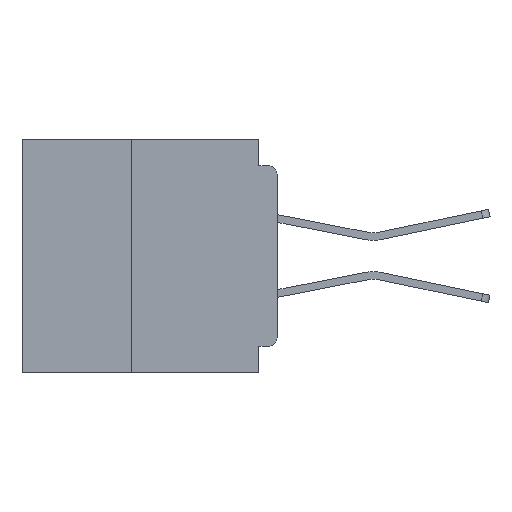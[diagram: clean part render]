
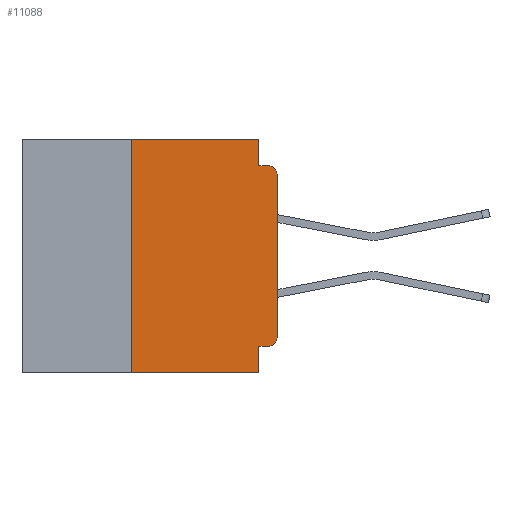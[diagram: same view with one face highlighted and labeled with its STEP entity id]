
A CAD part, left-side view. The second image highlights one B-rep face of the part: STEP entity #11088.
In plain terms, the highlighted planar face has unit normal (-1, 0, 0).
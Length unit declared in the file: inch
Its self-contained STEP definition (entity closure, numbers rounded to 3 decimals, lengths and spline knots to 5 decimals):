
#416 = VECTOR ( 'NONE', #36442, 39.37008 ) ;
#723 = ORIENTED_EDGE ( 'NONE', *, *, #28216, .F. ) ;
#1905 = VECTOR ( 'NONE', #16392, 39.37008 ) ;
#2743 = CARTESIAN_POINT ( 'NONE',  ( 0., 0., -0.06 ) ) ;
#3767 = VERTEX_POINT ( 'NONE', #39235 ) ;
#3960 = LINE ( 'NONE', #8334, #25589 ) ;
#4336 = AXIS2_PLACEMENT_3D ( 'NONE', #12253, #34526, #15499 ) ;
#4358 = EDGE_CURVE ( 'NONE', #33013, #12814, #26104, .T. ) ;
#5211 = CARTESIAN_POINT ( 'NONE',  ( 0., 0.031, -0.045 ) ) ;
#5717 = EDGE_CURVE ( 'NONE', #39130, #32010, #34941, .T. ) ;
#6209 = DIRECTION ( 'NONE',  ( -1., 0., 0. ) ) ;
#6236 = FACE_OUTER_BOUND ( 'NONE', #22828, .T. ) ;
#6773 = DIRECTION ( 'NONE',  ( 0., -1., 0. ) ) ;
#6792 = CARTESIAN_POINT ( 'NONE',  ( 0., 0.031, 0. ) ) ;
#6910 = CARTESIAN_POINT ( 'NONE',  ( 0., 0., -0.355 ) ) ;
#6939 = DIRECTION ( 'NONE',  ( 0., 0., -1. ) ) ;
#7150 = CARTESIAN_POINT ( 'NONE',  ( 0., 0.031, 0. ) ) ;
#7178 = ORIENTED_EDGE ( 'NONE', *, *, #34622, .F. ) ;
#7690 = VECTOR ( 'NONE', #29350, 39.37008 ) ;
#8334 = CARTESIAN_POINT ( 'NONE',  ( 0., 0., 0. ) ) ;
#8445 = VERTEX_POINT ( 'NONE', #33562 ) ;
#9411 = ORIENTED_EDGE ( 'NONE', *, *, #15265, .F. ) ;
#10151 = LINE ( 'NONE', #35265, #41008 ) ;
#10516 = CARTESIAN_POINT ( 'NONE',  ( 0., 0.031, -0.4 ) ) ;
#10726 = VECTOR ( 'NONE', #38511, 39.37008 ) ;
#11088 = ADVANCED_FACE ( 'NONE', ( #6236 ), #16538, .F. ) ;
#12033 = ORIENTED_EDGE ( 'NONE', *, *, #33776, .T. ) ;
#12253 = CARTESIAN_POINT ( 'NONE',  ( 0., 0.015, -0.06 ) ) ;
#12814 = VERTEX_POINT ( 'NONE', #13329 ) ;
#13329 = CARTESIAN_POINT ( 'NONE',  ( 0., 0.25, 0. ) ) ;
#13517 = DIRECTION ( 'NONE',  ( 0., -1., 0. ) ) ;
#14062 = CARTESIAN_POINT ( 'NONE',  ( 0., 0.25, -0.4 ) ) ;
#14987 = ORIENTED_EDGE ( 'NONE', *, *, #4358, .F. ) ;
#15265 = EDGE_CURVE ( 'NONE', #12814, #39130, #19229, .T. ) ;
#15499 = DIRECTION ( 'NONE',  ( 0., 0., -1. ) ) ;
#15989 = LINE ( 'NONE', #16206, #23517 ) ;
#16206 = CARTESIAN_POINT ( 'NONE',  ( 0., 0.031, -0.4 ) ) ;
#16341 = DIRECTION ( 'NONE',  ( 0., 0., -1. ) ) ;
#16392 = DIRECTION ( 'NONE',  ( 0., 0., -1. ) ) ;
#16538 = PLANE ( 'NONE',  #23182 ) ;
#17288 = LINE ( 'NONE', #6910, #7690 ) ;
#17349 = VERTEX_POINT ( 'NONE', #34319 ) ;
#19229 = LINE ( 'NONE', #35338, #10726 ) ;
#20596 = CARTESIAN_POINT ( 'NONE',  ( 0., 0.25, -0.4 ) ) ;
#21818 = CARTESIAN_POINT ( 'NONE',  ( 0., 0., -0.34 ) ) ;
#22828 = EDGE_LOOP ( 'NONE', ( #12033, #38961, #723, #23902, #9411, #14987, #37861, #7178, #33308, #24567 ) ) ;
#22988 = CARTESIAN_POINT ( 'NONE',  ( 0., 0.437, 0. ) ) ;
#23100 = EDGE_CURVE ( 'NONE', #17349, #27999, #38564, .T. ) ;
#23182 = AXIS2_PLACEMENT_3D ( 'NONE', #22988, #26183, #6939 ) ;
#23228 = EDGE_CURVE ( 'NONE', #33013, #26997, #10151, .T. ) ;
#23517 = VECTOR ( 'NONE', #16341, 39.37008 ) ;
#23902 = ORIENTED_EDGE ( 'NONE', *, *, #5717, .F. ) ;
#24482 = CIRCLE ( 'NONE', #4336, 0.015 ) ;
#24567 = ORIENTED_EDGE ( 'NONE', *, *, #23100, .T. ) ;
#25474 = CARTESIAN_POINT ( 'NONE',  ( 0., 0.015, -0.34 ) ) ;
#25589 = VECTOR ( 'NONE', #36937, 39.37008 ) ;
#26104 = LINE ( 'NONE', #14062, #416 ) ;
#26183 = DIRECTION ( 'NONE',  ( 1., 0., 0. ) ) ;
#26702 = VERTEX_POINT ( 'NONE', #2743 ) ;
#26997 = VERTEX_POINT ( 'NONE', #10516 ) ;
#27999 = VERTEX_POINT ( 'NONE', #21818 ) ;
#28181 = VECTOR ( 'NONE', #13517, 39.37008 ) ;
#28216 = EDGE_CURVE ( 'NONE', #32010, #3767, #31146, .T. ) ;
#28660 = DIRECTION ( 'NONE',  ( 0., 0., -1. ) ) ;
#29350 = DIRECTION ( 'NONE',  ( 0., 1., 0. ) ) ;
#30054 = AXIS2_PLACEMENT_3D ( 'NONE', #25474, #6209, #28660 ) ;
#31146 = LINE ( 'NONE', #38942, #28181 ) ;
#32010 = VERTEX_POINT ( 'NONE', #5211 ) ;
#33013 = VERTEX_POINT ( 'NONE', #20596 ) ;
#33308 = ORIENTED_EDGE ( 'NONE', *, *, #38476, .F. ) ;
#33562 = CARTESIAN_POINT ( 'NONE',  ( 0., 0.031, -0.355 ) ) ;
#33776 = EDGE_CURVE ( 'NONE', #27999, #26702, #3960, .T. ) ;
#34319 = CARTESIAN_POINT ( 'NONE',  ( 0., 0.015, -0.355 ) ) ;
#34526 = DIRECTION ( 'NONE',  ( -1., 0., 0. ) ) ;
#34622 = EDGE_CURVE ( 'NONE', #8445, #26997, #15989, .T. ) ;
#34941 = LINE ( 'NONE', #6792, #1905 ) ;
#35034 = EDGE_CURVE ( 'NONE', #26702, #3767, #24482, .T. ) ;
#35265 = CARTESIAN_POINT ( 'NONE',  ( 0., 0.437, -0.4 ) ) ;
#35338 = CARTESIAN_POINT ( 'NONE',  ( 0., 0.437, 0. ) ) ;
#36442 = DIRECTION ( 'NONE',  ( 0., 0., 1. ) ) ;
#36937 = DIRECTION ( 'NONE',  ( 0., 0., 1. ) ) ;
#37861 = ORIENTED_EDGE ( 'NONE', *, *, #23228, .T. ) ;
#38476 = EDGE_CURVE ( 'NONE', #17349, #8445, #17288, .T. ) ;
#38511 = DIRECTION ( 'NONE',  ( 0., -1., 0. ) ) ;
#38564 = CIRCLE ( 'NONE', #30054, 0.015 ) ;
#38942 = CARTESIAN_POINT ( 'NONE',  ( 0., 0., -0.045 ) ) ;
#38961 = ORIENTED_EDGE ( 'NONE', *, *, #35034, .T. ) ;
#39130 = VERTEX_POINT ( 'NONE', #7150 ) ;
#39235 = CARTESIAN_POINT ( 'NONE',  ( 0., 0.015, -0.045 ) ) ;
#41008 = VECTOR ( 'NONE', #6773, 39.37008 ) ;
